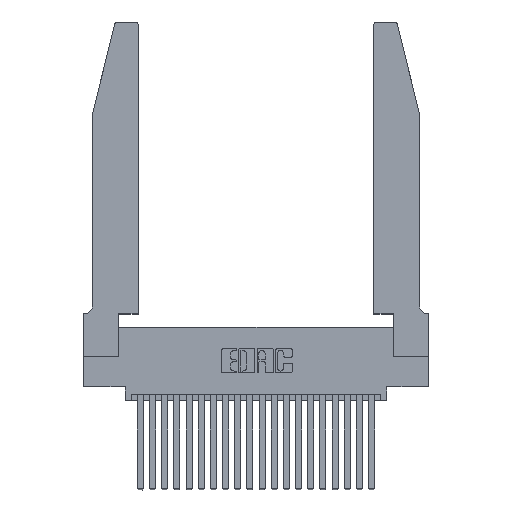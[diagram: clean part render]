
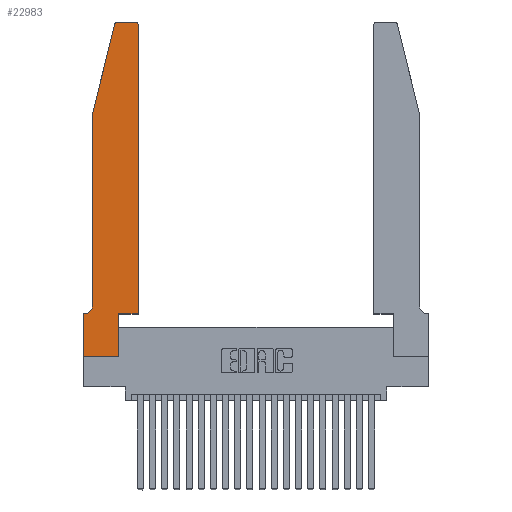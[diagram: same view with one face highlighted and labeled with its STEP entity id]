
A CAD part, top view. The second image highlights one B-rep face of the part: STEP entity #22983.
In plain terms, the highlighted planar face has unit normal (0, 0, 1).
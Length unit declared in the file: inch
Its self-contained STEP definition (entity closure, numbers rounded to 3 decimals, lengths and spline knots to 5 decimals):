
#49 = CARTESIAN_POINT ( 'NONE',  ( 0.25487, 2.72718, 0.37 ) ) ;
#131 = FACE_OUTER_BOUND ( 'NONE', #10386, .T. ) ;
#717 = ORIENTED_EDGE ( 'NONE', *, *, #12196, .T. ) ;
#925 = VERTEX_POINT ( 'NONE', #6084 ) ;
#1061 = CARTESIAN_POINT ( 'NONE',  ( 0.0755, 0.35, 0.37 ) ) ;
#1205 = CARTESIAN_POINT ( 'NONE',  ( 0.0755, 2., 0.37 ) ) ;
#1471 = VECTOR ( 'NONE', #18588, 39.37008 ) ;
#1619 = EDGE_CURVE ( 'NONE', #6916, #18420, #12518, .T. ) ;
#1802 = VERTEX_POINT ( 'NONE', #8434 ) ;
#2695 = DIRECTION ( 'NONE',  ( 0., 1., 0. ) ) ;
#3524 = CARTESIAN_POINT ( 'NONE',  ( 0.4505, 0.35, 0.37 ) ) ;
#3821 = DIRECTION ( 'NONE',  ( 0., -1., 0. ) ) ;
#4023 = VECTOR ( 'NONE', #4258, 39.37008 ) ;
#4126 = ORIENTED_EDGE ( 'NONE', *, *, #6508, .T. ) ;
#4163 = VECTOR ( 'NONE', #13716, 39.37008 ) ;
#4258 = DIRECTION ( 'NONE',  ( 1., 0., 0. ) ) ;
#4483 = VERTEX_POINT ( 'NONE', #14396 ) ;
#4672 = LINE ( 'NONE', #11684, #10012 ) ;
#4755 = DIRECTION ( 'NONE',  ( 0., 0., -1. ) ) ;
#5320 = DIRECTION ( 'NONE',  ( -1., 0., 0. ) ) ;
#5873 = VERTEX_POINT ( 'NONE', #17007 ) ;
#6004 = CARTESIAN_POINT ( 'NONE',  ( 0.0755, 2., 0.37 ) ) ;
#6018 = ORIENTED_EDGE ( 'NONE', *, *, #10642, .T. ) ;
#6084 = CARTESIAN_POINT ( 'NONE',  ( 0.2865, 0.35, 0.37 ) ) ;
#6134 = DIRECTION ( 'NONE',  ( 1., 0., 0. ) ) ;
#6508 = EDGE_CURVE ( 'NONE', #4483, #14214, #18904, .T. ) ;
#6916 = VERTEX_POINT ( 'NONE', #49 ) ;
#7026 = CARTESIAN_POINT ( 'NONE',  ( 0.284, 2.72, 0.37 ) ) ;
#7217 = ORIENTED_EDGE ( 'NONE', *, *, #1619, .T. ) ;
#7278 = ORIENTED_EDGE ( 'NONE', *, *, #10728, .T. ) ;
#7306 = CARTESIAN_POINT ( 'NONE',  ( 0.2605, 2.75, 0.37 ) ) ;
#7520 = AXIS2_PLACEMENT_3D ( 'NONE', #17011, #16935, #6134 ) ;
#7577 = CIRCLE ( 'NONE', #7520, 0.03 ) ;
#8221 = LINE ( 'NONE', #14191, #17256 ) ;
#8227 = CARTESIAN_POINT ( 'NONE',  ( 0., 0.35, 0.37 ) ) ;
#8300 = DIRECTION ( 'NONE',  ( -1., 0., 0. ) ) ;
#8351 = ORIENTED_EDGE ( 'NONE', *, *, #19470, .T. ) ;
#8434 = CARTESIAN_POINT ( 'NONE',  ( 0.4505, 2.72, 0.37 ) ) ;
#8854 = VECTOR ( 'NONE', #2695, 39.37008 ) ;
#9270 = CARTESIAN_POINT ( 'NONE',  ( 0.0755, 2., 0.37 ) ) ;
#9542 = CARTESIAN_POINT ( 'NONE',  ( 0.2865, 0., 0.37 ) ) ;
#9722 = LINE ( 'NONE', #7306, #11668 ) ;
#9843 = EDGE_CURVE ( 'NONE', #11527, #22864, #9722, .T. ) ;
#9931 = ORIENTED_EDGE ( 'NONE', *, *, #16075, .T. ) ;
#10012 = VECTOR ( 'NONE', #21257, 39.37008 ) ;
#10386 = EDGE_LOOP ( 'NONE', ( #20834, #7278, #7217, #6018, #4126, #717, #8351, #15738, #12672, #9931, #19699, #19271 ) ) ;
#10538 = EDGE_CURVE ( 'NONE', #5873, #15722, #19813, .T. ) ;
#10547 = CARTESIAN_POINT ( 'NONE',  ( 0.4505, 0.35, 0.37 ) ) ;
#10642 = EDGE_CURVE ( 'NONE', #18420, #4483, #13643, .T. ) ;
#10728 = EDGE_CURVE ( 'NONE', #22864, #6916, #20098, .T. ) ;
#10878 = CARTESIAN_POINT ( 'NONE',  ( 0.4205, 2.75, 0.37 ) ) ;
#11527 = VERTEX_POINT ( 'NONE', #10878 ) ;
#11668 = VECTOR ( 'NONE', #5320, 39.37008 ) ;
#11684 = CARTESIAN_POINT ( 'NONE',  ( 0.4505, 0.35, 0.37 ) ) ;
#11830 = PLANE ( 'NONE',  #21790 ) ;
#12196 = EDGE_CURVE ( 'NONE', #14214, #19897, #21391, .T. ) ;
#12199 = DIRECTION ( 'NONE',  ( 0., 0., 1. ) ) ;
#12216 = LINE ( 'NONE', #13596, #8854 ) ;
#12518 = LINE ( 'NONE', #6004, #1471 ) ;
#12672 = ORIENTED_EDGE ( 'NONE', *, *, #18815, .T. ) ;
#13230 = CARTESIAN_POINT ( 'NONE',  ( 0., 0.35, 0.37 ) ) ;
#13596 = CARTESIAN_POINT ( 'NONE',  ( 0.2865, 0.35, 0.37 ) ) ;
#13643 = LINE ( 'NONE', #1205, #15025 ) ;
#13711 = DIRECTION ( 'NONE',  ( 0., -1., 0. ) ) ;
#13716 = DIRECTION ( 'NONE',  ( -1., 0., 0. ) ) ;
#14191 = CARTESIAN_POINT ( 'NONE',  ( 0., 0., 0.37 ) ) ;
#14214 = VERTEX_POINT ( 'NONE', #22634 ) ;
#14257 = DIRECTION ( 'NONE',  ( 1., 0., 0. ) ) ;
#14396 = CARTESIAN_POINT ( 'NONE',  ( 0.0755, 0.42, 0.37 ) ) ;
#15025 = VECTOR ( 'NONE', #13711, 39.37008 ) ;
#15111 = AXIS2_PLACEMENT_3D ( 'NONE', #7026, #12199, #14257 ) ;
#15722 = VERTEX_POINT ( 'NONE', #9542 ) ;
#15738 = ORIENTED_EDGE ( 'NONE', *, *, #10538, .T. ) ;
#15904 = AXIS2_PLACEMENT_3D ( 'NONE', #18868, #4755, #8300 ) ;
#16075 = EDGE_CURVE ( 'NONE', #925, #22619, #21509, .T. ) ;
#16919 = CARTESIAN_POINT ( 'NONE',  ( 0.284, 2.75, 0.37 ) ) ;
#16935 = DIRECTION ( 'NONE',  ( 0., 0., 1. ) ) ;
#17007 = CARTESIAN_POINT ( 'NONE',  ( 0., 0., 0.37 ) ) ;
#17011 = CARTESIAN_POINT ( 'NONE',  ( 0.4205, 2.72, 0.37 ) ) ;
#17256 = VECTOR ( 'NONE', #3821, 39.37008 ) ;
#18065 = EDGE_CURVE ( 'NONE', #1802, #11527, #7577, .T. ) ;
#18272 = EDGE_CURVE ( 'NONE', #22619, #1802, #4672, .T. ) ;
#18420 = VERTEX_POINT ( 'NONE', #9270 ) ;
#18588 = DIRECTION ( 'NONE',  ( -0.239, -0.971, 0. ) ) ;
#18815 = EDGE_CURVE ( 'NONE', #15722, #925, #12216, .T. ) ;
#18851 = CARTESIAN_POINT ( 'NONE',  ( 0., 0., 0.37 ) ) ;
#18868 = CARTESIAN_POINT ( 'NONE',  ( 0.0055, 0.42, 0.37 ) ) ;
#18904 = CIRCLE ( 'NONE', #15904, 0.07 ) ;
#19271 = ORIENTED_EDGE ( 'NONE', *, *, #18065, .T. ) ;
#19373 = DIRECTION ( 'NONE',  ( 1., 0., 0. ) ) ;
#19470 = EDGE_CURVE ( 'NONE', #19897, #5873, #8221, .T. ) ;
#19699 = ORIENTED_EDGE ( 'NONE', *, *, #18272, .T. ) ;
#19790 = VECTOR ( 'NONE', #19373, 39.37008 ) ;
#19813 = LINE ( 'NONE', #18851, #4023 ) ;
#19897 = VERTEX_POINT ( 'NONE', #13230 ) ;
#20098 = CIRCLE ( 'NONE', #15111, 0.03 ) ;
#20733 = DIRECTION ( 'NONE',  ( 0., 0., 1. ) ) ;
#20834 = ORIENTED_EDGE ( 'NONE', *, *, #9843, .T. ) ;
#21257 = DIRECTION ( 'NONE',  ( 0., 1., 0. ) ) ;
#21391 = LINE ( 'NONE', #1061, #4163 ) ;
#21509 = LINE ( 'NONE', #10547, #19790 ) ;
#21790 = AXIS2_PLACEMENT_3D ( 'NONE', #8227, #20733, #22661 ) ;
#22619 = VERTEX_POINT ( 'NONE', #3524 ) ;
#22634 = CARTESIAN_POINT ( 'NONE',  ( 0.0055, 0.35, 0.37 ) ) ;
#22661 = DIRECTION ( 'NONE',  ( 1., 0., 0. ) ) ;
#22864 = VERTEX_POINT ( 'NONE', #16919 ) ;
#22983 = ADVANCED_FACE ( 'NONE', ( #131 ), #11830, .T. ) ;
